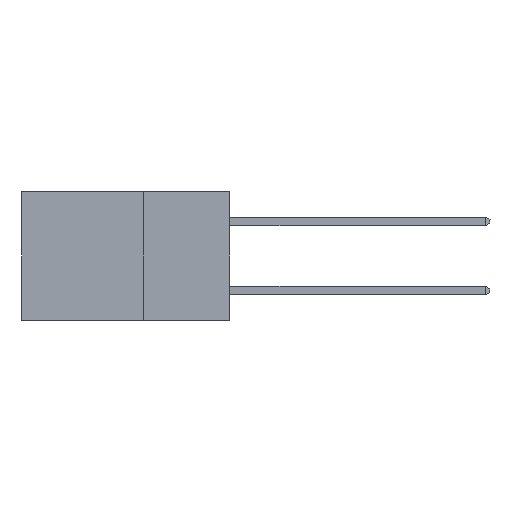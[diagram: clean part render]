
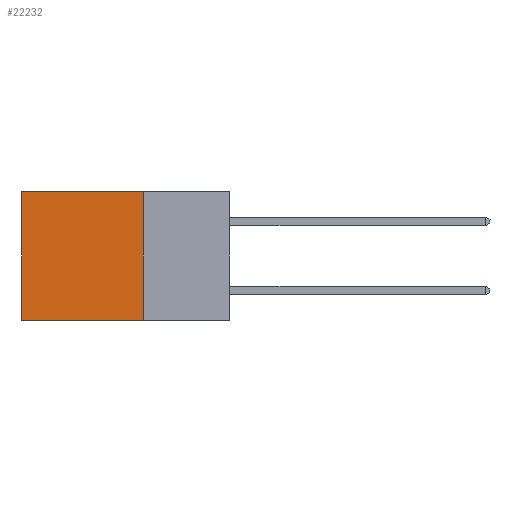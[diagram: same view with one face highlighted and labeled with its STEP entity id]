
A CAD part, left-side view. The second image highlights one B-rep face of the part: STEP entity #22232.
In plain terms, the highlighted planar face has unit normal (-1, 0, 0).
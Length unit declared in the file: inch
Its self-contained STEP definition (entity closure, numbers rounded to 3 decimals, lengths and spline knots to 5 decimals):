
#211 = VECTOR ( 'NONE', #2522, 39.37008 ) ;
#764 = AXIS2_PLACEMENT_3D ( 'NONE', #13425, #29063, #15681 ) ;
#2522 = DIRECTION ( 'NONE',  ( 0., 0., -1. ) ) ;
#4412 = VERTEX_POINT ( 'NONE', #28525 ) ;
#4857 = CARTESIAN_POINT ( 'NONE',  ( 0.298, 0.6, 0. ) ) ;
#5654 = ORIENTED_EDGE ( 'NONE', *, *, #7217, .T. ) ;
#6945 = CARTESIAN_POINT ( 'NONE',  ( 0.298, 0.25, -0.37 ) ) ;
#7217 = EDGE_CURVE ( 'NONE', #4412, #13035, #12346, .T. ) ;
#8658 = CARTESIAN_POINT ( 'NONE',  ( 0.298, 0.25, -0.37 ) ) ;
#10374 = LINE ( 'NONE', #20974, #15636 ) ;
#10852 = ORIENTED_EDGE ( 'NONE', *, *, #19755, .F. ) ;
#12212 = EDGE_CURVE ( 'NONE', #22454, #4412, #10374, .T. ) ;
#12346 = LINE ( 'NONE', #4857, #211 ) ;
#13035 = VERTEX_POINT ( 'NONE', #25796 ) ;
#13182 = FACE_OUTER_BOUND ( 'NONE', #14726, .T. ) ;
#13249 = PLANE ( 'NONE',  #764 ) ;
#13315 = DIRECTION ( 'NONE',  ( 0., 0., -1. ) ) ;
#13425 = CARTESIAN_POINT ( 'NONE',  ( 0.298, 0.25, 0. ) ) ;
#13756 = ORIENTED_EDGE ( 'NONE', *, *, #26149, .F. ) ;
#14726 = EDGE_LOOP ( 'NONE', ( #5654, #13756, #10852, #16723 ) ) ;
#15636 = VECTOR ( 'NONE', #18079, 39.37008 ) ;
#15681 = DIRECTION ( 'NONE',  ( 0., 0., -1. ) ) ;
#16723 = ORIENTED_EDGE ( 'NONE', *, *, #12212, .T. ) ;
#17189 = VECTOR ( 'NONE', #27209, 39.37008 ) ;
#18079 = DIRECTION ( 'NONE',  ( 0., 1., 0. ) ) ;
#18625 = CARTESIAN_POINT ( 'NONE',  ( 0.298, 0.25, 0. ) ) ;
#19393 = VECTOR ( 'NONE', #13315, 39.37008 ) ;
#19755 = EDGE_CURVE ( 'NONE', #22454, #28974, #20091, .T. ) ;
#19990 = CARTESIAN_POINT ( 'NONE',  ( 0.298, 0.25, 0. ) ) ;
#20091 = LINE ( 'NONE', #19990, #19393 ) ;
#20974 = CARTESIAN_POINT ( 'NONE',  ( 0.298, 0.25, 0. ) ) ;
#22232 = ADVANCED_FACE ( 'NONE', ( #13182 ), #13249, .F. ) ;
#22454 = VERTEX_POINT ( 'NONE', #18625 ) ;
#23881 = LINE ( 'NONE', #6945, #17189 ) ;
#25796 = CARTESIAN_POINT ( 'NONE',  ( 0.298, 0.6, -0.37 ) ) ;
#26149 = EDGE_CURVE ( 'NONE', #28974, #13035, #23881, .T. ) ;
#27209 = DIRECTION ( 'NONE',  ( 0., 1., 0. ) ) ;
#28525 = CARTESIAN_POINT ( 'NONE',  ( 0.298, 0.6, 0. ) ) ;
#28974 = VERTEX_POINT ( 'NONE', #8658 ) ;
#29063 = DIRECTION ( 'NONE',  ( 1., 0., 0. ) ) ;
